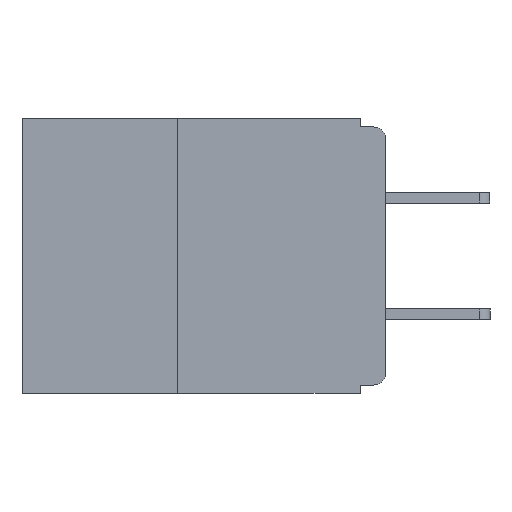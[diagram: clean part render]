
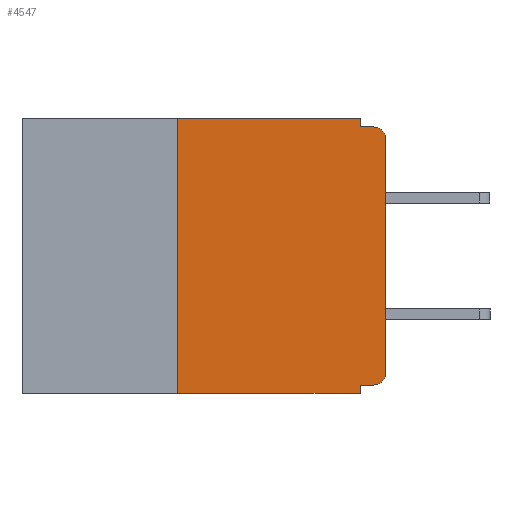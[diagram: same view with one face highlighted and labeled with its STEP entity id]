
A CAD part, left-side view. The second image highlights one B-rep face of the part: STEP entity #4547.
In plain terms, the highlighted planar face has unit normal (-1, 0, 0).
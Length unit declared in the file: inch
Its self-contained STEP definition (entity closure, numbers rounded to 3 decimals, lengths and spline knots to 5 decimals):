
#18 = CARTESIAN_POINT ( 'NONE',  ( 0., 0., -0.305 ) ) ;
#3013 = EDGE_CURVE ( 'NONE', #19683, #23217, #25303, .T. ) ;
#3055 = EDGE_CURVE ( 'NONE', #16423, #24575, #16802, .T. ) ;
#3309 = CARTESIAN_POINT ( 'NONE',  ( 0., 0.25, -0.33 ) ) ;
#3346 = LINE ( 'NONE', #6505, #16533 ) ;
#3561 = VERTEX_POINT ( 'NONE', #18 ) ;
#3568 = ORIENTED_EDGE ( 'NONE', *, *, #28432, .T. ) ;
#4547 = ADVANCED_FACE ( 'NONE', ( #10957 ), #6669, .F. ) ;
#4766 = DIRECTION ( 'NONE',  ( 0., -1., 0. ) ) ;
#5343 = EDGE_CURVE ( 'NONE', #23217, #20076, #8880, .T. ) ;
#5358 = LINE ( 'NONE', #13165, #19306 ) ;
#5782 = EDGE_CURVE ( 'NONE', #20076, #24575, #15807, .T. ) ;
#5909 = CARTESIAN_POINT ( 'NONE',  ( 0., 0., -0.025 ) ) ;
#5924 = VERTEX_POINT ( 'NONE', #19330 ) ;
#6113 = VECTOR ( 'NONE', #24363, 39.37008 ) ;
#6131 = CARTESIAN_POINT ( 'NONE',  ( 0., 0.437, 0. ) ) ;
#6505 = CARTESIAN_POINT ( 'NONE',  ( 0., 0., 0. ) ) ;
#6516 = ORIENTED_EDGE ( 'NONE', *, *, #22943, .F. ) ;
#6624 = DIRECTION ( 'NONE',  ( 0., 0., 1. ) ) ;
#6669 = PLANE ( 'NONE',  #11315 ) ;
#6736 = VECTOR ( 'NONE', #15510, 39.37008 ) ;
#8200 = AXIS2_PLACEMENT_3D ( 'NONE', #30663, #15296, #33130 ) ;
#8633 = EDGE_LOOP ( 'NONE', ( #3568, #31971, #12286, #26849, #33509, #20829, #28446, #24856, #6516, #14346 ) ) ;
#8880 = LINE ( 'NONE', #29729, #15057 ) ;
#8896 = EDGE_CURVE ( 'NONE', #19004, #14556, #20778, .T. ) ;
#10957 = FACE_OUTER_BOUND ( 'NONE', #8633, .T. ) ;
#11315 = AXIS2_PLACEMENT_3D ( 'NONE', #6131, #13800, #20613 ) ;
#11329 = EDGE_CURVE ( 'NONE', #24635, #14556, #20657, .T. ) ;
#11500 = VECTOR ( 'NONE', #4766, 39.37008 ) ;
#12286 = ORIENTED_EDGE ( 'NONE', *, *, #5782, .F. ) ;
#12808 = CIRCLE ( 'NONE', #8200, 0.015 ) ;
#12867 = CARTESIAN_POINT ( 'NONE',  ( 0., 0.015, -0.01 ) ) ;
#13165 = CARTESIAN_POINT ( 'NONE',  ( 0., 0., -0.32 ) ) ;
#13231 = EDGE_CURVE ( 'NONE', #5924, #3561, #12808, .T. ) ;
#13357 = DIRECTION ( 'NONE',  ( -1., 0., 0. ) ) ;
#13800 = DIRECTION ( 'NONE',  ( 1., 0., 0. ) ) ;
#14346 = ORIENTED_EDGE ( 'NONE', *, *, #13231, .T. ) ;
#14556 = VERTEX_POINT ( 'NONE', #29339 ) ;
#15057 = VECTOR ( 'NONE', #29558, 39.37008 ) ;
#15296 = DIRECTION ( 'NONE',  ( -1., 0., 0. ) ) ;
#15510 = DIRECTION ( 'NONE',  ( 0., 0., -1. ) ) ;
#15807 = LINE ( 'NONE', #24091, #22709 ) ;
#15884 = CARTESIAN_POINT ( 'NONE',  ( 0., 0.015, -0.025 ) ) ;
#16423 = VERTEX_POINT ( 'NONE', #5909 ) ;
#16533 = VECTOR ( 'NONE', #6624, 39.37008 ) ;
#16802 = CIRCLE ( 'NONE', #18060, 0.015 ) ;
#17119 = EDGE_CURVE ( 'NONE', #19004, #19683, #26888, .T. ) ;
#17657 = CARTESIAN_POINT ( 'NONE',  ( 0., 0.031, -0.01 ) ) ;
#17975 = CARTESIAN_POINT ( 'NONE',  ( 0., 0.031, -0.33 ) ) ;
#18060 = AXIS2_PLACEMENT_3D ( 'NONE', #15884, #13357, #18977 ) ;
#18457 = DIRECTION ( 'NONE',  ( 0., 1., 0. ) ) ;
#18977 = DIRECTION ( 'NONE',  ( 0., 0., -1. ) ) ;
#19004 = VERTEX_POINT ( 'NONE', #30964 ) ;
#19306 = VECTOR ( 'NONE', #18457, 39.37008 ) ;
#19330 = CARTESIAN_POINT ( 'NONE',  ( 0., 0.015, -0.32 ) ) ;
#19683 = VERTEX_POINT ( 'NONE', #31585 ) ;
#20076 = VERTEX_POINT ( 'NONE', #17657 ) ;
#20613 = DIRECTION ( 'NONE',  ( 0., 0., -1. ) ) ;
#20657 = LINE ( 'NONE', #17975, #6736 ) ;
#20778 = LINE ( 'NONE', #23673, #25998 ) ;
#20829 = ORIENTED_EDGE ( 'NONE', *, *, #17119, .F. ) ;
#22709 = VECTOR ( 'NONE', #23864, 39.37008 ) ;
#22943 = EDGE_CURVE ( 'NONE', #5924, #24635, #5358, .T. ) ;
#23217 = VERTEX_POINT ( 'NONE', #30154 ) ;
#23673 = CARTESIAN_POINT ( 'NONE',  ( 0., 0.437, -0.33 ) ) ;
#23864 = DIRECTION ( 'NONE',  ( 0., -1., 0. ) ) ;
#24091 = CARTESIAN_POINT ( 'NONE',  ( 0., 0., -0.01 ) ) ;
#24363 = DIRECTION ( 'NONE',  ( 0., 0., 1. ) ) ;
#24575 = VERTEX_POINT ( 'NONE', #12867 ) ;
#24635 = VERTEX_POINT ( 'NONE', #33539 ) ;
#24856 = ORIENTED_EDGE ( 'NONE', *, *, #11329, .F. ) ;
#25303 = LINE ( 'NONE', #29348, #11500 ) ;
#25998 = VECTOR ( 'NONE', #28835, 39.37008 ) ;
#26849 = ORIENTED_EDGE ( 'NONE', *, *, #5343, .F. ) ;
#26888 = LINE ( 'NONE', #3309, #6113 ) ;
#28432 = EDGE_CURVE ( 'NONE', #3561, #16423, #3346, .T. ) ;
#28446 = ORIENTED_EDGE ( 'NONE', *, *, #8896, .T. ) ;
#28835 = DIRECTION ( 'NONE',  ( 0., -1., 0. ) ) ;
#29339 = CARTESIAN_POINT ( 'NONE',  ( 0., 0.031, -0.33 ) ) ;
#29348 = CARTESIAN_POINT ( 'NONE',  ( 0., 0.437, 0. ) ) ;
#29558 = DIRECTION ( 'NONE',  ( 0., 0., -1. ) ) ;
#29729 = CARTESIAN_POINT ( 'NONE',  ( 0., 0.031, 0. ) ) ;
#30154 = CARTESIAN_POINT ( 'NONE',  ( 0., 0.031, 0. ) ) ;
#30663 = CARTESIAN_POINT ( 'NONE',  ( 0., 0.015, -0.305 ) ) ;
#30964 = CARTESIAN_POINT ( 'NONE',  ( 0., 0.25, -0.33 ) ) ;
#31585 = CARTESIAN_POINT ( 'NONE',  ( 0., 0.25, 0. ) ) ;
#31971 = ORIENTED_EDGE ( 'NONE', *, *, #3055, .T. ) ;
#33130 = DIRECTION ( 'NONE',  ( 0., 0., -1. ) ) ;
#33509 = ORIENTED_EDGE ( 'NONE', *, *, #3013, .F. ) ;
#33539 = CARTESIAN_POINT ( 'NONE',  ( 0., 0.031, -0.32 ) ) ;
